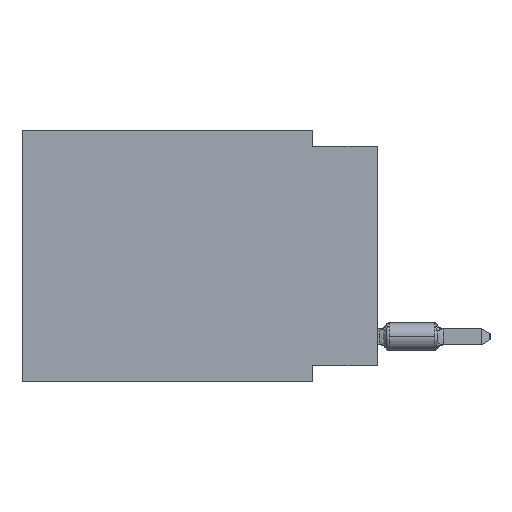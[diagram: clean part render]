
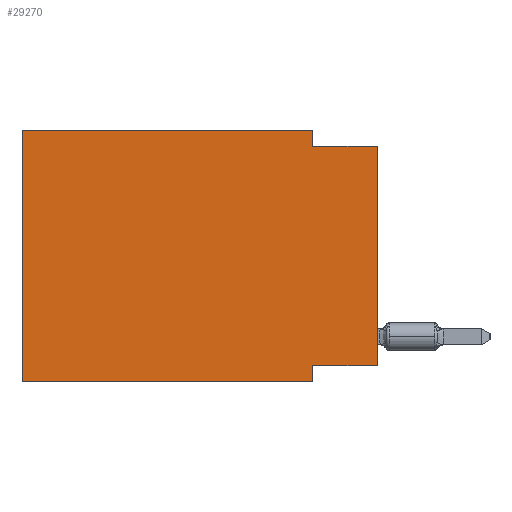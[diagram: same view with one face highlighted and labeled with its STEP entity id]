
A CAD part, left-side view. The second image highlights one B-rep face of the part: STEP entity #29270.
In plain terms, the highlighted planar face has unit normal (-1, 0, 0).
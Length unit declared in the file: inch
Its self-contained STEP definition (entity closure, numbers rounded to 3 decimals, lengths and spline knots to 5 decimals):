
#1259 = VERTEX_POINT ( 'NONE', #40188 ) ;
#1743 = VERTEX_POINT ( 'NONE', #5856 ) ;
#3504 = ORIENTED_EDGE ( 'NONE', *, *, #17015, .T. ) ;
#4641 = CARTESIAN_POINT ( 'NONE',  ( 0., 0., -0.365 ) ) ;
#5806 = CARTESIAN_POINT ( 'NONE',  ( 0., 0.55, 0. ) ) ;
#5856 = CARTESIAN_POINT ( 'NONE',  ( 0., 0.1, 0. ) ) ;
#6103 = VECTOR ( 'NONE', #36400, 39.37008 ) ;
#6495 = CARTESIAN_POINT ( 'NONE',  ( 0., 0.1, -0.39 ) ) ;
#6919 = EDGE_CURVE ( 'NONE', #1743, #37238, #39680, .T. ) ;
#7538 = DIRECTION ( 'NONE',  ( 0., 1., 0. ) ) ;
#7582 = EDGE_CURVE ( 'NONE', #38953, #22642, #35795, .T. ) ;
#7700 = LINE ( 'NONE', #27662, #17426 ) ;
#8615 = EDGE_LOOP ( 'NONE', ( #3504, #20608, #10333, #29752, #25261, #35208, #9654, #16280 ) ) ;
#8998 = DIRECTION ( 'NONE',  ( 0., 0., -1. ) ) ;
#9654 = ORIENTED_EDGE ( 'NONE', *, *, #37311, .F. ) ;
#9877 = CARTESIAN_POINT ( 'NONE',  ( 0., 0.1, 0. ) ) ;
#10136 = VECTOR ( 'NONE', #42360, 39.37008 ) ;
#10333 = ORIENTED_EDGE ( 'NONE', *, *, #6919, .F. ) ;
#11991 = DIRECTION ( 'NONE',  ( 0., -1., 0. ) ) ;
#12428 = LINE ( 'NONE', #36608, #6103 ) ;
#12581 = DIRECTION ( 'NONE',  ( 0., 0., 1. ) ) ;
#14889 = VECTOR ( 'NONE', #11991, 39.37008 ) ;
#15719 = EDGE_CURVE ( 'NONE', #1259, #39986, #35439, .T. ) ;
#15776 = LINE ( 'NONE', #33258, #14889 ) ;
#16280 = ORIENTED_EDGE ( 'NONE', *, *, #7582, .F. ) ;
#16376 = CARTESIAN_POINT ( 'NONE',  ( 0., 0.1, -0.025 ) ) ;
#16575 = CARTESIAN_POINT ( 'NONE',  ( 0., 0.1, -0.365 ) ) ;
#17015 = EDGE_CURVE ( 'NONE', #38953, #24746, #29588, .T. ) ;
#17386 = CARTESIAN_POINT ( 'NONE',  ( 0., 0.55, 0. ) ) ;
#17426 = VECTOR ( 'NONE', #35283, 39.37008 ) ;
#17647 = CARTESIAN_POINT ( 'NONE',  ( 0., 0.1, -0.39 ) ) ;
#18827 = VECTOR ( 'NONE', #12581, 39.37008 ) ;
#19097 = CARTESIAN_POINT ( 'NONE',  ( 0., 0., -0.365 ) ) ;
#19354 = VECTOR ( 'NONE', #8998, 39.37008 ) ;
#20608 = ORIENTED_EDGE ( 'NONE', *, *, #35510, .F. ) ;
#20621 = DIRECTION ( 'NONE',  ( 0., 0., -1. ) ) ;
#21784 = CARTESIAN_POINT ( 'NONE',  ( 0., 0., -0.025 ) ) ;
#22642 = VERTEX_POINT ( 'NONE', #16575 ) ;
#24514 = EDGE_CURVE ( 'NONE', #39986, #1743, #15776, .T. ) ;
#24746 = VERTEX_POINT ( 'NONE', #21784 ) ;
#25261 = ORIENTED_EDGE ( 'NONE', *, *, #15719, .F. ) ;
#26424 = DIRECTION ( 'NONE',  ( 0., 0., -1. ) ) ;
#26466 = AXIS2_PLACEMENT_3D ( 'NONE', #5806, #27290, #26424 ) ;
#27290 = DIRECTION ( 'NONE',  ( 1., 0., 0. ) ) ;
#27662 = CARTESIAN_POINT ( 'NONE',  ( 0., 0., -0.025 ) ) ;
#28359 = VERTEX_POINT ( 'NONE', #17647 ) ;
#28690 = CARTESIAN_POINT ( 'NONE',  ( 0., 0.55, 0. ) ) ;
#29270 = ADVANCED_FACE ( 'NONE', ( #44094 ), #40307, .F. ) ;
#29588 = LINE ( 'NONE', #43251, #18827 ) ;
#29752 = ORIENTED_EDGE ( 'NONE', *, *, #24514, .F. ) ;
#30414 = VECTOR ( 'NONE', #20621, 39.37008 ) ;
#33258 = CARTESIAN_POINT ( 'NONE',  ( 0., 0.55, 0. ) ) ;
#35208 = ORIENTED_EDGE ( 'NONE', *, *, #37914, .T. ) ;
#35283 = DIRECTION ( 'NONE',  ( 0., -1., 0. ) ) ;
#35439 = LINE ( 'NONE', #28690, #10136 ) ;
#35510 = EDGE_CURVE ( 'NONE', #37238, #24746, #7700, .T. ) ;
#35795 = LINE ( 'NONE', #4641, #41632 ) ;
#36400 = DIRECTION ( 'NONE',  ( 0., -1., 0. ) ) ;
#36608 = CARTESIAN_POINT ( 'NONE',  ( 0., 0.55, -0.39 ) ) ;
#37238 = VERTEX_POINT ( 'NONE', #16376 ) ;
#37311 = EDGE_CURVE ( 'NONE', #22642, #28359, #37415, .T. ) ;
#37415 = LINE ( 'NONE', #6495, #30414 ) ;
#37914 = EDGE_CURVE ( 'NONE', #1259, #28359, #12428, .T. ) ;
#38953 = VERTEX_POINT ( 'NONE', #19097 ) ;
#39680 = LINE ( 'NONE', #9877, #19354 ) ;
#39986 = VERTEX_POINT ( 'NONE', #17386 ) ;
#40188 = CARTESIAN_POINT ( 'NONE',  ( 0., 0.55, -0.39 ) ) ;
#40307 = PLANE ( 'NONE',  #26466 ) ;
#41632 = VECTOR ( 'NONE', #7538, 39.37008 ) ;
#42360 = DIRECTION ( 'NONE',  ( 0., 0., 1. ) ) ;
#43251 = CARTESIAN_POINT ( 'NONE',  ( 0., 0., 0. ) ) ;
#44094 = FACE_OUTER_BOUND ( 'NONE', #8615, .T. ) ;
